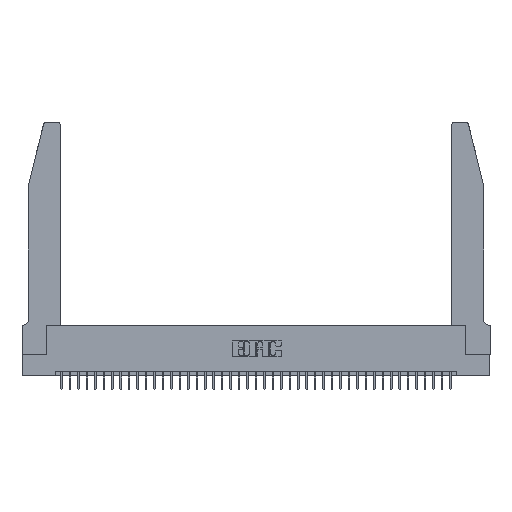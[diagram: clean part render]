
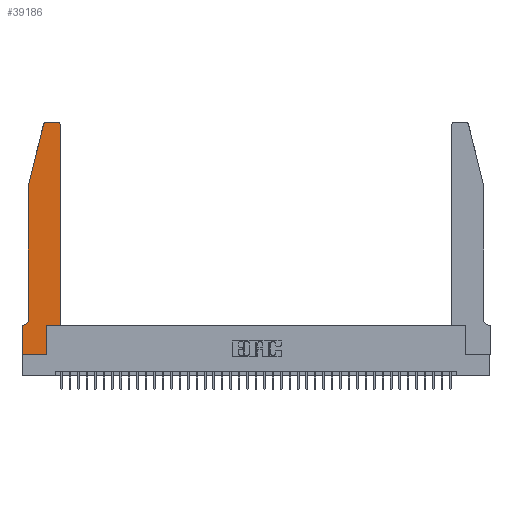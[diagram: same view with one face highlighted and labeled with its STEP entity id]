
A CAD part, top view. The second image highlights one B-rep face of the part: STEP entity #39186.
In plain terms, the highlighted planar face has unit normal (0, 0, 1).
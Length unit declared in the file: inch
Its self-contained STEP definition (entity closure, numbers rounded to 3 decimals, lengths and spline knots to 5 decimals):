
#52 = EDGE_CURVE ( 'NONE', #22433, #38477, #8196, .T. ) ;
#598 = DIRECTION ( 'NONE',  ( -1., 0., 0. ) ) ;
#1618 = CARTESIAN_POINT ( 'NONE',  ( 0.4505, 2.72, 0.37 ) ) ;
#2158 = ORIENTED_EDGE ( 'NONE', *, *, #2583, .T. ) ;
#2559 = DIRECTION ( 'NONE',  ( 1., 0., 0. ) ) ;
#2583 = EDGE_CURVE ( 'NONE', #7594, #22433, #32353, .T. ) ;
#2807 = DIRECTION ( 'NONE',  ( 1., 0., 0. ) ) ;
#2831 = DIRECTION ( 'NONE',  ( 0., 0., 1. ) ) ;
#3272 = LINE ( 'NONE', #15712, #10640 ) ;
#3642 = VECTOR ( 'NONE', #28848, 39.37008 ) ;
#3836 = CIRCLE ( 'NONE', #4142, 0.03 ) ;
#3949 = CARTESIAN_POINT ( 'NONE',  ( 0., 0., 0.37 ) ) ;
#4142 = AXIS2_PLACEMENT_3D ( 'NONE', #27712, #2831, #2559 ) ;
#4620 = FACE_OUTER_BOUND ( 'NONE', #16292, .T. ) ;
#4995 = EDGE_CURVE ( 'NONE', #9306, #20835, #8143, .T. ) ;
#5029 = DIRECTION ( 'NONE',  ( 1., 0., 0. ) ) ;
#5480 = CARTESIAN_POINT ( 'NONE',  ( 0.0055, 0.35, 0.37 ) ) ;
#5566 = ORIENTED_EDGE ( 'NONE', *, *, #15928, .T. ) ;
#5974 = CARTESIAN_POINT ( 'NONE',  ( 0., 0., 0.37 ) ) ;
#7594 = VERTEX_POINT ( 'NONE', #24815 ) ;
#7652 = VECTOR ( 'NONE', #10866, 39.37008 ) ;
#7728 = ORIENTED_EDGE ( 'NONE', *, *, #12429, .T. ) ;
#8143 = CIRCLE ( 'NONE', #22061, 0.03 ) ;
#8150 = VERTEX_POINT ( 'NONE', #9699 ) ;
#8196 = LINE ( 'NONE', #33739, #40971 ) ;
#8431 = ORIENTED_EDGE ( 'NONE', *, *, #19081, .T. ) ;
#8485 = VECTOR ( 'NONE', #19602, 39.37008 ) ;
#9306 = VERTEX_POINT ( 'NONE', #1618 ) ;
#9621 = CIRCLE ( 'NONE', #35384, 0.07 ) ;
#9699 = CARTESIAN_POINT ( 'NONE',  ( 0.4505, 0.35, 0.37 ) ) ;
#10088 = LINE ( 'NONE', #5974, #10621 ) ;
#10370 = ORIENTED_EDGE ( 'NONE', *, *, #30162, .T. ) ;
#10621 = VECTOR ( 'NONE', #2807, 39.37008 ) ;
#10640 = VECTOR ( 'NONE', #598, 39.37008 ) ;
#10866 = DIRECTION ( 'NONE',  ( 0., 1., 0. ) ) ;
#10867 = LINE ( 'NONE', #3949, #34223 ) ;
#11495 = EDGE_CURVE ( 'NONE', #32540, #18816, #35297, .T. ) ;
#11795 = VECTOR ( 'NONE', #5029, 39.37008 ) ;
#12088 = DIRECTION ( 'NONE',  ( 0., 0., -1. ) ) ;
#12429 = EDGE_CURVE ( 'NONE', #37893, #21203, #10867, .T. ) ;
#14051 = LINE ( 'NONE', #17214, #7652 ) ;
#14149 = DIRECTION ( 'NONE',  ( 0., -1., 0. ) ) ;
#15246 = DIRECTION ( 'NONE',  ( -1., 0., 0. ) ) ;
#15402 = DIRECTION ( 'NONE',  ( 0., 0., 1. ) ) ;
#15453 = CARTESIAN_POINT ( 'NONE',  ( 0.0755, 0.42, 0.37 ) ) ;
#15491 = CARTESIAN_POINT ( 'NONE',  ( 0.0755, 2., 0.37 ) ) ;
#15712 = CARTESIAN_POINT ( 'NONE',  ( 0.2605, 2.75, 0.37 ) ) ;
#15928 = EDGE_CURVE ( 'NONE', #21203, #32540, #10088, .T. ) ;
#16292 = EDGE_LOOP ( 'NONE', ( #21867, #37040, #2158, #19475, #40584, #8431, #7728, #5566, #26911, #10370, #34760, #34006 ) ) ;
#16454 = CARTESIAN_POINT ( 'NONE',  ( 0.2865, 0.35, 0.37 ) ) ;
#16482 = CARTESIAN_POINT ( 'NONE',  ( 0.0755, 2., 0.37 ) ) ;
#17214 = CARTESIAN_POINT ( 'NONE',  ( 0.4505, 0.35, 0.37 ) ) ;
#18382 = VERTEX_POINT ( 'NONE', #36271 ) ;
#18816 = VERTEX_POINT ( 'NONE', #39599 ) ;
#18911 = CARTESIAN_POINT ( 'NONE',  ( 0.0755, 0.35, 0.37 ) ) ;
#19081 = EDGE_CURVE ( 'NONE', #27777, #37893, #19859, .T. ) ;
#19475 = ORIENTED_EDGE ( 'NONE', *, *, #52, .T. ) ;
#19602 = DIRECTION ( 'NONE',  ( 0., 1., 0. ) ) ;
#19859 = LINE ( 'NONE', #18911, #21863 ) ;
#20835 = VERTEX_POINT ( 'NONE', #38385 ) ;
#21184 = CARTESIAN_POINT ( 'NONE',  ( 0.4205, 2.72, 0.37 ) ) ;
#21203 = VERTEX_POINT ( 'NONE', #32275 ) ;
#21863 = VECTOR ( 'NONE', #22080, 39.37008 ) ;
#21867 = ORIENTED_EDGE ( 'NONE', *, *, #31967, .T. ) ;
#22061 = AXIS2_PLACEMENT_3D ( 'NONE', #21184, #32283, #25837 ) ;
#22080 = DIRECTION ( 'NONE',  ( -1., 0., 0. ) ) ;
#22433 = VERTEX_POINT ( 'NONE', #15491 ) ;
#22441 = EDGE_CURVE ( 'NONE', #18382, #7594, #3836, .T. ) ;
#24175 = LINE ( 'NONE', #26185, #11795 ) ;
#24815 = CARTESIAN_POINT ( 'NONE',  ( 0.25487, 2.72718, 0.37 ) ) ;
#25837 = DIRECTION ( 'NONE',  ( 1., 0., 0. ) ) ;
#26185 = CARTESIAN_POINT ( 'NONE',  ( 0.4505, 0.35, 0.37 ) ) ;
#26911 = ORIENTED_EDGE ( 'NONE', *, *, #11495, .T. ) ;
#27090 = EDGE_CURVE ( 'NONE', #8150, #9306, #14051, .T. ) ;
#27712 = CARTESIAN_POINT ( 'NONE',  ( 0.284, 2.72, 0.37 ) ) ;
#27777 = VERTEX_POINT ( 'NONE', #5480 ) ;
#28067 = AXIS2_PLACEMENT_3D ( 'NONE', #34456, #15402, #37640 ) ;
#28449 = PLANE ( 'NONE',  #28067 ) ;
#28848 = DIRECTION ( 'NONE',  ( -0.239, -0.971, 0. ) ) ;
#30162 = EDGE_CURVE ( 'NONE', #18816, #8150, #24175, .T. ) ;
#31099 = CARTESIAN_POINT ( 'NONE',  ( 0.0055, 0.42, 0.37 ) ) ;
#31967 = EDGE_CURVE ( 'NONE', #20835, #18382, #3272, .T. ) ;
#32275 = CARTESIAN_POINT ( 'NONE',  ( 0., 0., 0.37 ) ) ;
#32283 = DIRECTION ( 'NONE',  ( 0., 0., 1. ) ) ;
#32353 = LINE ( 'NONE', #16482, #3642 ) ;
#32482 = EDGE_CURVE ( 'NONE', #38477, #27777, #9621, .T. ) ;
#32483 = DIRECTION ( 'NONE',  ( 0., -1., 0. ) ) ;
#32540 = VERTEX_POINT ( 'NONE', #38018 ) ;
#33739 = CARTESIAN_POINT ( 'NONE',  ( 0.0755, 2., 0.37 ) ) ;
#34006 = ORIENTED_EDGE ( 'NONE', *, *, #4995, .T. ) ;
#34223 = VECTOR ( 'NONE', #32483, 39.37008 ) ;
#34456 = CARTESIAN_POINT ( 'NONE',  ( 0., 0.35, 0.37 ) ) ;
#34760 = ORIENTED_EDGE ( 'NONE', *, *, #27090, .T. ) ;
#35297 = LINE ( 'NONE', #16454, #8485 ) ;
#35384 = AXIS2_PLACEMENT_3D ( 'NONE', #31099, #12088, #15246 ) ;
#36271 = CARTESIAN_POINT ( 'NONE',  ( 0.284, 2.75, 0.37 ) ) ;
#37040 = ORIENTED_EDGE ( 'NONE', *, *, #22441, .T. ) ;
#37640 = DIRECTION ( 'NONE',  ( 1., 0., 0. ) ) ;
#37893 = VERTEX_POINT ( 'NONE', #40940 ) ;
#38018 = CARTESIAN_POINT ( 'NONE',  ( 0.2865, 0., 0.37 ) ) ;
#38385 = CARTESIAN_POINT ( 'NONE',  ( 0.4205, 2.75, 0.37 ) ) ;
#38477 = VERTEX_POINT ( 'NONE', #15453 ) ;
#39186 = ADVANCED_FACE ( 'NONE', ( #4620 ), #28449, .T. ) ;
#39599 = CARTESIAN_POINT ( 'NONE',  ( 0.2865, 0.35, 0.37 ) ) ;
#40584 = ORIENTED_EDGE ( 'NONE', *, *, #32482, .T. ) ;
#40940 = CARTESIAN_POINT ( 'NONE',  ( 0., 0.35, 0.37 ) ) ;
#40971 = VECTOR ( 'NONE', #14149, 39.37008 ) ;
